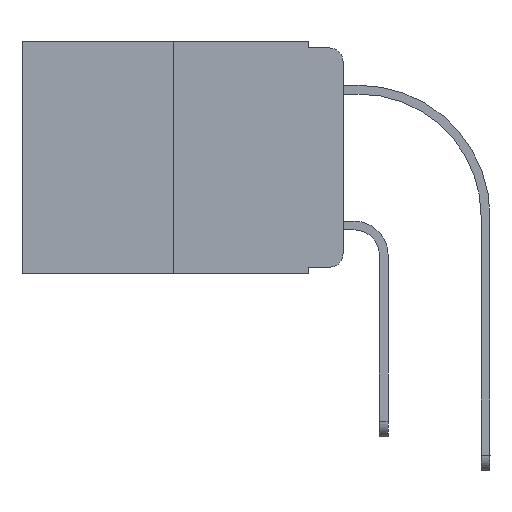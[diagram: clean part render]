
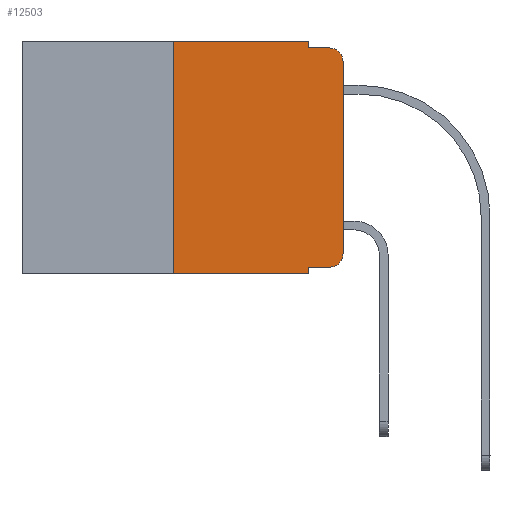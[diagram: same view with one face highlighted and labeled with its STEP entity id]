
A CAD part, left-side view. The second image highlights one B-rep face of the part: STEP entity #12503.
In plain terms, the highlighted planar face has unit normal (-1, 0, 0).
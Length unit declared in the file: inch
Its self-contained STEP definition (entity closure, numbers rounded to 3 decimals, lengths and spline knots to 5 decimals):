
#106 = CARTESIAN_POINT ( 'NONE',  ( 0., 0., 0. ) ) ;
#522 = VECTOR ( 'NONE', #18797, 39.37008 ) ;
#804 = ORIENTED_EDGE ( 'NONE', *, *, #4881, .F. ) ;
#896 = AXIS2_PLACEMENT_3D ( 'NONE', #2920, #4558, #6316 ) ;
#1098 = LINE ( 'NONE', #3208, #5501 ) ;
#1214 = DIRECTION ( 'NONE',  ( 0., -1., 0. ) ) ;
#1289 = CARTESIAN_POINT ( 'NONE',  ( 0., 0.473, -0.343 ) ) ;
#1442 = CARTESIAN_POINT ( 'NONE',  ( 0., 0.25, 0. ) ) ;
#1911 = CARTESIAN_POINT ( 'NONE',  ( 0., 0.051, -0.333 ) ) ;
#2056 = ORIENTED_EDGE ( 'NONE', *, *, #12026, .F. ) ;
#2310 = ORIENTED_EDGE ( 'NONE', *, *, #22769, .T. ) ;
#2626 = VECTOR ( 'NONE', #14169, 39.37008 ) ;
#2920 = CARTESIAN_POINT ( 'NONE',  ( 0., 0.473, 0. ) ) ;
#3196 = ORIENTED_EDGE ( 'NONE', *, *, #20091, .T. ) ;
#3208 = CARTESIAN_POINT ( 'NONE',  ( 0., 0.051, -0.01 ) ) ;
#3356 = LINE ( 'NONE', #5455, #19330 ) ;
#3460 = CIRCLE ( 'NONE', #16178, 0.02 ) ;
#3700 = CARTESIAN_POINT ( 'NONE',  ( 0., 0.051, -0.343 ) ) ;
#4249 = CARTESIAN_POINT ( 'NONE',  ( 0., 0.02, -0.333 ) ) ;
#4302 = VERTEX_POINT ( 'NONE', #16279 ) ;
#4558 = DIRECTION ( 'NONE',  ( 1., 0., 0. ) ) ;
#4576 = DIRECTION ( 'NONE',  ( 0., 0., -1. ) ) ;
#4600 = EDGE_LOOP ( 'NONE', ( #16986, #3196, #10209, #804, #2056, #7036, #2310, #22392, #8324, #11605 ) ) ;
#4697 = LINE ( 'NONE', #1289, #21165 ) ;
#4881 = EDGE_CURVE ( 'NONE', #4302, #21845, #12620, .T. ) ;
#5038 = CIRCLE ( 'NONE', #6177, 0.02 ) ;
#5455 = CARTESIAN_POINT ( 'NONE',  ( 0., 0.051, 0. ) ) ;
#5501 = VECTOR ( 'NONE', #1214, 39.37008 ) ;
#5614 = EDGE_CURVE ( 'NONE', #18612, #21252, #19666, .T. ) ;
#6005 = EDGE_CURVE ( 'NONE', #19813, #14599, #3356, .T. ) ;
#6177 = AXIS2_PLACEMENT_3D ( 'NONE', #17240, #15467, #4576 ) ;
#6316 = DIRECTION ( 'NONE',  ( 0., 0., -1. ) ) ;
#6548 = DIRECTION ( 'NONE',  ( 0., 0., 1. ) ) ;
#6719 = VERTEX_POINT ( 'NONE', #4249 ) ;
#6848 = CARTESIAN_POINT ( 'NONE',  ( 0., 0.051, -0.01 ) ) ;
#7036 = ORIENTED_EDGE ( 'NONE', *, *, #7290, .F. ) ;
#7290 = EDGE_CURVE ( 'NONE', #15908, #17120, #22138, .T. ) ;
#7674 = CARTESIAN_POINT ( 'NONE',  ( 0., 0.051, 0. ) ) ;
#8324 = ORIENTED_EDGE ( 'NONE', *, *, #13646, .T. ) ;
#9271 = CARTESIAN_POINT ( 'NONE',  ( 0., 0., -0.313 ) ) ;
#9685 = VERTEX_POINT ( 'NONE', #17823 ) ;
#10209 = ORIENTED_EDGE ( 'NONE', *, *, #10338, .F. ) ;
#10338 = EDGE_CURVE ( 'NONE', #21845, #9685, #1098, .T. ) ;
#10479 = DIRECTION ( 'NONE',  ( 0., -1., 0. ) ) ;
#10627 = DIRECTION ( 'NONE',  ( 0., 0., -1. ) ) ;
#11586 = DIRECTION ( 'NONE',  ( 0., 0., -1. ) ) ;
#11605 = ORIENTED_EDGE ( 'NONE', *, *, #20526, .T. ) ;
#11830 = FACE_OUTER_BOUND ( 'NONE', #4600, .T. ) ;
#12026 = EDGE_CURVE ( 'NONE', #17120, #4302, #16936, .T. ) ;
#12503 = ADVANCED_FACE ( 'NONE', ( #11830 ), #15446, .F. ) ;
#12620 = LINE ( 'NONE', #7674, #12621 ) ;
#12621 = VECTOR ( 'NONE', #13073, 39.37008 ) ;
#13073 = DIRECTION ( 'NONE',  ( 0., 0., -1. ) ) ;
#13580 = CARTESIAN_POINT ( 'NONE',  ( 0., 0.02, -0.313 ) ) ;
#13646 = EDGE_CURVE ( 'NONE', #19813, #6719, #21133, .T. ) ;
#13838 = DIRECTION ( 'NONE',  ( 0., -1., 0. ) ) ;
#14169 = DIRECTION ( 'NONE',  ( 0., 0., 1. ) ) ;
#14599 = VERTEX_POINT ( 'NONE', #3700 ) ;
#15446 = PLANE ( 'NONE',  #896 ) ;
#15453 = CARTESIAN_POINT ( 'NONE',  ( 0., 0.25, 0. ) ) ;
#15467 = DIRECTION ( 'NONE',  ( -1., 0., 0. ) ) ;
#15713 = CARTESIAN_POINT ( 'NONE',  ( 0., 0.473, 0. ) ) ;
#15908 = VERTEX_POINT ( 'NONE', #17808 ) ;
#16178 = AXIS2_PLACEMENT_3D ( 'NONE', #13580, #16867, #11586 ) ;
#16197 = CARTESIAN_POINT ( 'NONE',  ( 0., 0.051, -0.333 ) ) ;
#16279 = CARTESIAN_POINT ( 'NONE',  ( 0., 0.051, 0. ) ) ;
#16508 = VECTOR ( 'NONE', #6548, 39.37008 ) ;
#16867 = DIRECTION ( 'NONE',  ( -1., 0., 0. ) ) ;
#16936 = LINE ( 'NONE', #15713, #522 ) ;
#16986 = ORIENTED_EDGE ( 'NONE', *, *, #5614, .T. ) ;
#17120 = VERTEX_POINT ( 'NONE', #1442 ) ;
#17240 = CARTESIAN_POINT ( 'NONE',  ( 0., 0.02, -0.03 ) ) ;
#17808 = CARTESIAN_POINT ( 'NONE',  ( 0., 0.25, -0.343 ) ) ;
#17823 = CARTESIAN_POINT ( 'NONE',  ( 0., 0.02, -0.01 ) ) ;
#18140 = VECTOR ( 'NONE', #10479, 39.37008 ) ;
#18612 = VERTEX_POINT ( 'NONE', #9271 ) ;
#18797 = DIRECTION ( 'NONE',  ( 0., -1., 0. ) ) ;
#19330 = VECTOR ( 'NONE', #10627, 39.37008 ) ;
#19666 = LINE ( 'NONE', #106, #2626 ) ;
#19813 = VERTEX_POINT ( 'NONE', #16197 ) ;
#20091 = EDGE_CURVE ( 'NONE', #21252, #9685, #5038, .T. ) ;
#20526 = EDGE_CURVE ( 'NONE', #6719, #18612, #3460, .T. ) ;
#20596 = CARTESIAN_POINT ( 'NONE',  ( 0., 0., -0.03 ) ) ;
#21133 = LINE ( 'NONE', #1911, #18140 ) ;
#21165 = VECTOR ( 'NONE', #13838, 39.37008 ) ;
#21252 = VERTEX_POINT ( 'NONE', #20596 ) ;
#21845 = VERTEX_POINT ( 'NONE', #6848 ) ;
#22138 = LINE ( 'NONE', #15453, #16508 ) ;
#22392 = ORIENTED_EDGE ( 'NONE', *, *, #6005, .F. ) ;
#22769 = EDGE_CURVE ( 'NONE', #15908, #14599, #4697, .T. ) ;
